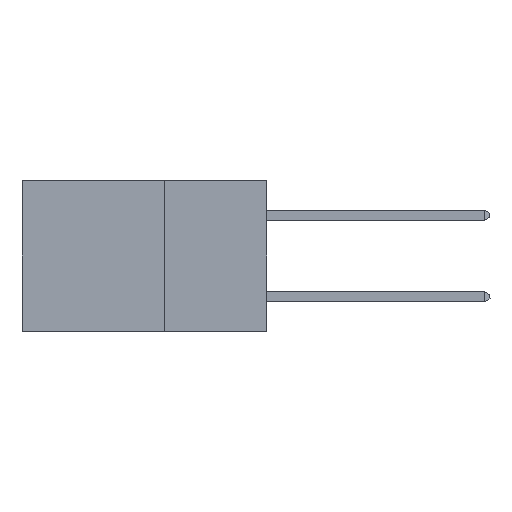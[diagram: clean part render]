
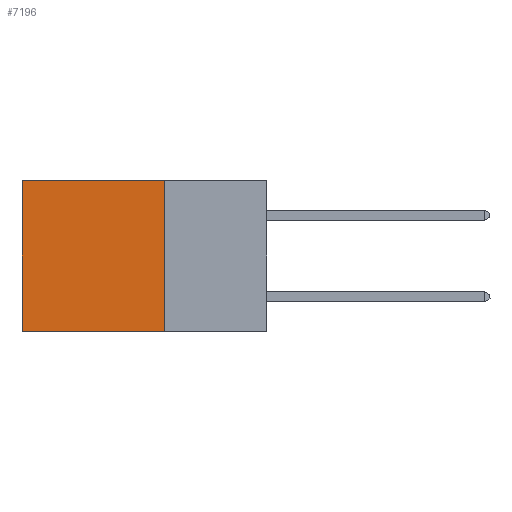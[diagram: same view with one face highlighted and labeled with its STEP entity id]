
A CAD part, left-side view. The second image highlights one B-rep face of the part: STEP entity #7196.
In plain terms, the highlighted planar face has unit normal (-1, 0, 0).
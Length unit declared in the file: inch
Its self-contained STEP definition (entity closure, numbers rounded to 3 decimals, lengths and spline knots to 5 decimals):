
#326 = CARTESIAN_POINT ( 'NONE',  ( 0.2875, 0.25, 0. ) ) ;
#398 = VECTOR ( 'NONE', #11595, 39.37008 ) ;
#914 = DIRECTION ( 'NONE',  ( 0., 1., 0. ) ) ;
#996 = CARTESIAN_POINT ( 'NONE',  ( 0.2875, 0.25, 0. ) ) ;
#1746 = FACE_OUTER_BOUND ( 'NONE', #2179, .T. ) ;
#1753 = DIRECTION ( 'NONE',  ( 1., 0., 0. ) ) ;
#2179 = EDGE_LOOP ( 'NONE', ( #19014, #12582, #6286, #9446 ) ) ;
#2209 = CARTESIAN_POINT ( 'NONE',  ( 0.2875, 0.6, -0.37 ) ) ;
#2478 = DIRECTION ( 'NONE',  ( 0., 1., 0. ) ) ;
#2625 = CARTESIAN_POINT ( 'NONE',  ( 0.2875, 0.25, 0. ) ) ;
#3121 = LINE ( 'NONE', #17632, #18129 ) ;
#5346 = CARTESIAN_POINT ( 'NONE',  ( 0.2875, 0.25, -0.37 ) ) ;
#6286 = ORIENTED_EDGE ( 'NONE', *, *, #6402, .F. ) ;
#6402 = EDGE_CURVE ( 'NONE', #17748, #10627, #19319, .T. ) ;
#6876 = EDGE_CURVE ( 'NONE', #17748, #6914, #8272, .T. ) ;
#6914 = VERTEX_POINT ( 'NONE', #7011 ) ;
#7011 = CARTESIAN_POINT ( 'NONE',  ( 0.2875, 0.6, 0. ) ) ;
#7196 = ADVANCED_FACE ( 'NONE', ( #1746 ), #10723, .F. ) ;
#7589 = EDGE_CURVE ( 'NONE', #6914, #19273, #3121, .T. ) ;
#7785 = VECTOR ( 'NONE', #2478, 39.37008 ) ;
#8272 = LINE ( 'NONE', #996, #7785 ) ;
#9446 = ORIENTED_EDGE ( 'NONE', *, *, #6876, .T. ) ;
#10627 = VERTEX_POINT ( 'NONE', #17305 ) ;
#10723 = PLANE ( 'NONE',  #14470 ) ;
#11595 = DIRECTION ( 'NONE',  ( 0., 0., -1. ) ) ;
#11992 = EDGE_CURVE ( 'NONE', #10627, #19273, #17016, .T. ) ;
#12251 = DIRECTION ( 'NONE',  ( 0., 0., -1. ) ) ;
#12582 = ORIENTED_EDGE ( 'NONE', *, *, #11992, .F. ) ;
#13554 = VECTOR ( 'NONE', #914, 39.37008 ) ;
#14470 = AXIS2_PLACEMENT_3D ( 'NONE', #15224, #1753, #12251 ) ;
#15224 = CARTESIAN_POINT ( 'NONE',  ( 0.2875, 0.25, 0. ) ) ;
#17016 = LINE ( 'NONE', #5346, #13554 ) ;
#17305 = CARTESIAN_POINT ( 'NONE',  ( 0.2875, 0.25, -0.37 ) ) ;
#17632 = CARTESIAN_POINT ( 'NONE',  ( 0.2875, 0.6, 0. ) ) ;
#17748 = VERTEX_POINT ( 'NONE', #326 ) ;
#18129 = VECTOR ( 'NONE', #19127, 39.37008 ) ;
#19014 = ORIENTED_EDGE ( 'NONE', *, *, #7589, .T. ) ;
#19127 = DIRECTION ( 'NONE',  ( 0., 0., -1. ) ) ;
#19273 = VERTEX_POINT ( 'NONE', #2209 ) ;
#19319 = LINE ( 'NONE', #2625, #398 ) ;
